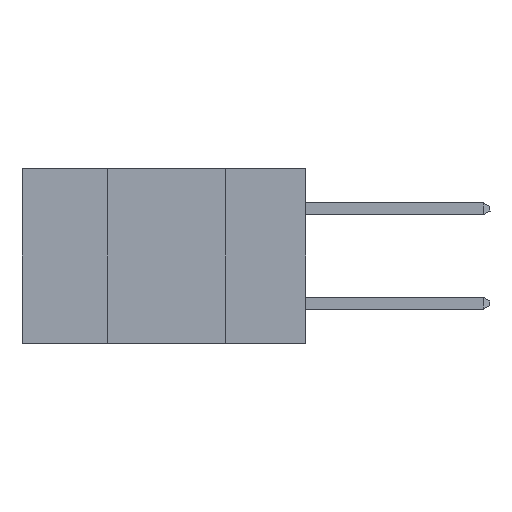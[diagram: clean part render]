
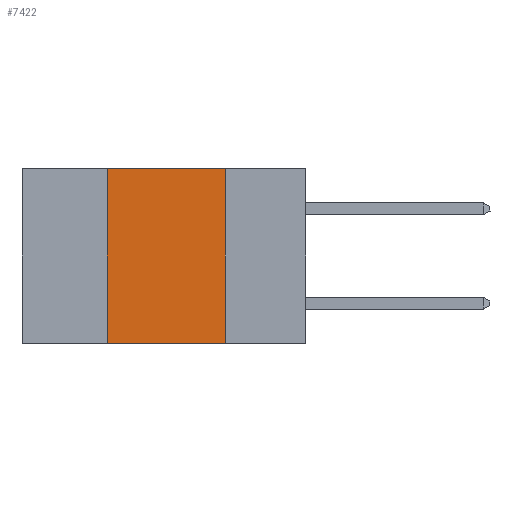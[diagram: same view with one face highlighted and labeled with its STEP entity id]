
A CAD part, left-side view. The second image highlights one B-rep face of the part: STEP entity #7422.
In plain terms, the highlighted planar face has unit normal (-1, 0, 0).
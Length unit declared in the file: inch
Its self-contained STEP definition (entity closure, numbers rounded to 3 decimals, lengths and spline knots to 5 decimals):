
#85 = CARTESIAN_POINT ( 'NONE',  ( 0., 0.42, -0.37 ) ) ;
#379 = ORIENTED_EDGE ( 'NONE', *, *, #14478, .T. ) ;
#428 = VERTEX_POINT ( 'NONE', #13512 ) ;
#1318 = CARTESIAN_POINT ( 'NONE',  ( 0., 0.42, 0. ) ) ;
#1489 = DIRECTION ( 'NONE',  ( 0., 0., 1. ) ) ;
#2129 = VECTOR ( 'NONE', #24419, 39.37008 ) ;
#3308 = VECTOR ( 'NONE', #5128, 39.37008 ) ;
#4606 = VERTEX_POINT ( 'NONE', #85 ) ;
#4851 = ORIENTED_EDGE ( 'NONE', *, *, #8770, .F. ) ;
#5128 = DIRECTION ( 'NONE',  ( 0., 0., -1. ) ) ;
#5332 = EDGE_CURVE ( 'NONE', #428, #22354, #8338, .T. ) ;
#7422 = ADVANCED_FACE ( 'NONE', ( #15676 ), #16549, .F. ) ;
#8328 = EDGE_CURVE ( 'NONE', #22354, #16256, #13442, .T. ) ;
#8338 = LINE ( 'NONE', #17904, #2129 ) ;
#8770 = EDGE_CURVE ( 'NONE', #4606, #428, #16579, .T. ) ;
#9468 = CARTESIAN_POINT ( 'NONE',  ( 0., 0.17, 0. ) ) ;
#9728 = CARTESIAN_POINT ( 'NONE',  ( 0., 0.17, 0. ) ) ;
#10347 = EDGE_LOOP ( 'NONE', ( #11084, #22198, #4851, #379 ) ) ;
#11075 = VECTOR ( 'NONE', #1489, 39.37008 ) ;
#11084 = ORIENTED_EDGE ( 'NONE', *, *, #8328, .F. ) ;
#13339 = AXIS2_PLACEMENT_3D ( 'NONE', #18622, #19167, #20745 ) ;
#13442 = LINE ( 'NONE', #9468, #3308 ) ;
#13512 = CARTESIAN_POINT ( 'NONE',  ( 0., 0.42, 0. ) ) ;
#14478 = EDGE_CURVE ( 'NONE', #4606, #16256, #18980, .T. ) ;
#15676 = FACE_OUTER_BOUND ( 'NONE', #10347, .T. ) ;
#16256 = VERTEX_POINT ( 'NONE', #21505 ) ;
#16549 = PLANE ( 'NONE',  #13339 ) ;
#16579 = LINE ( 'NONE', #1318, #11075 ) ;
#17904 = CARTESIAN_POINT ( 'NONE',  ( 0., 0.6, 0. ) ) ;
#18622 = CARTESIAN_POINT ( 'NONE',  ( 0., 0.6, 0. ) ) ;
#18980 = LINE ( 'NONE', #19477, #19951 ) ;
#19167 = DIRECTION ( 'NONE',  ( 1., 0., 0. ) ) ;
#19477 = CARTESIAN_POINT ( 'NONE',  ( 0., 0.6, -0.37 ) ) ;
#19951 = VECTOR ( 'NONE', #21590, 39.37008 ) ;
#20745 = DIRECTION ( 'NONE',  ( 0., 0., -1. ) ) ;
#21505 = CARTESIAN_POINT ( 'NONE',  ( 0., 0.17, -0.37 ) ) ;
#21590 = DIRECTION ( 'NONE',  ( 0., -1., 0. ) ) ;
#22198 = ORIENTED_EDGE ( 'NONE', *, *, #5332, .F. ) ;
#22354 = VERTEX_POINT ( 'NONE', #9728 ) ;
#24419 = DIRECTION ( 'NONE',  ( 0., -1., 0. ) ) ;
